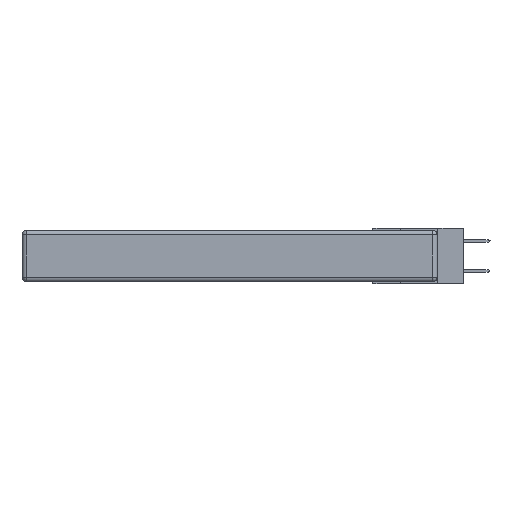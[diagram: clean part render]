
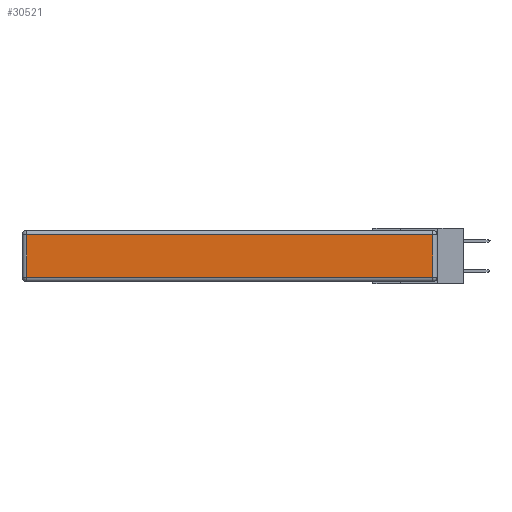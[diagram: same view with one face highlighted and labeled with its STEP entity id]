
A CAD part, left-side view. The second image highlights one B-rep face of the part: STEP entity #30521.
In plain terms, the highlighted planar face has unit normal (-1, 0, 0).
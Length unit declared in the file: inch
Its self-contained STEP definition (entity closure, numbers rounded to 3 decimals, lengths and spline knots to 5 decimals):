
#622 = ORIENTED_EDGE ( 'NONE', *, *, #10707, .T. ) ;
#784 = ORIENTED_EDGE ( 'NONE', *, *, #23932, .T. ) ;
#2432 = LINE ( 'NONE', #18635, #27938 ) ;
#3144 = CARTESIAN_POINT ( 'NONE',  ( 0., 2.72, -0.343 ) ) ;
#5120 = DIRECTION ( 'NONE',  ( 0., -1., 0. ) ) ;
#6020 = PLANE ( 'NONE',  #17279 ) ;
#6114 = DIRECTION ( 'NONE',  ( -1., 0., 0. ) ) ;
#7294 = FACE_OUTER_BOUND ( 'NONE', #12953, .T. ) ;
#8809 = LINE ( 'NONE', #15509, #21969 ) ;
#9784 = CARTESIAN_POINT ( 'NONE',  ( 0., 2.72, -0.313 ) ) ;
#9972 = LINE ( 'NONE', #3144, #15625 ) ;
#10502 = DIRECTION ( 'NONE',  ( 0., 0., -1. ) ) ;
#10707 = EDGE_CURVE ( 'NONE', #22136, #23475, #8809, .T. ) ;
#11506 = CARTESIAN_POINT ( 'NONE',  ( 0., 2.72, -0.03 ) ) ;
#11718 = LINE ( 'NONE', #29129, #13208 ) ;
#12953 = EDGE_LOOP ( 'NONE', ( #24868, #622, #18886, #784 ) ) ;
#13208 = VECTOR ( 'NONE', #5120, 39.37008 ) ;
#14981 = VERTEX_POINT ( 'NONE', #11506 ) ;
#15388 = DIRECTION ( 'NONE',  ( 0., 0., 1. ) ) ;
#15509 = CARTESIAN_POINT ( 'NONE',  ( 0., 0.03, -0.343 ) ) ;
#15625 = VECTOR ( 'NONE', #10502, 39.37008 ) ;
#16681 = EDGE_CURVE ( 'NONE', #27656, #22136, #11718, .T. ) ;
#17279 = AXIS2_PLACEMENT_3D ( 'NONE', #27632, #6114, #15388 ) ;
#17625 = DIRECTION ( 'NONE',  ( 0., 0., 1. ) ) ;
#18635 = CARTESIAN_POINT ( 'NONE',  ( 0., 2.75, -0.03 ) ) ;
#18886 = ORIENTED_EDGE ( 'NONE', *, *, #30579, .T. ) ;
#19116 = CARTESIAN_POINT ( 'NONE',  ( 0., 0.03, -0.03 ) ) ;
#21969 = VECTOR ( 'NONE', #17625, 39.37008 ) ;
#22136 = VERTEX_POINT ( 'NONE', #28108 ) ;
#23475 = VERTEX_POINT ( 'NONE', #19116 ) ;
#23932 = EDGE_CURVE ( 'NONE', #14981, #27656, #9972, .T. ) ;
#24868 = ORIENTED_EDGE ( 'NONE', *, *, #16681, .T. ) ;
#27632 = CARTESIAN_POINT ( 'NONE',  ( 0., 0., -0.343 ) ) ;
#27656 = VERTEX_POINT ( 'NONE', #9784 ) ;
#27938 = VECTOR ( 'NONE', #30206, 39.37008 ) ;
#28108 = CARTESIAN_POINT ( 'NONE',  ( 0., 0.03, -0.313 ) ) ;
#29129 = CARTESIAN_POINT ( 'NONE',  ( 0., 0., -0.313 ) ) ;
#30206 = DIRECTION ( 'NONE',  ( 0., 1., 0. ) ) ;
#30521 = ADVANCED_FACE ( 'NONE', ( #7294 ), #6020, .T. ) ;
#30579 = EDGE_CURVE ( 'NONE', #23475, #14981, #2432, .T. ) ;
